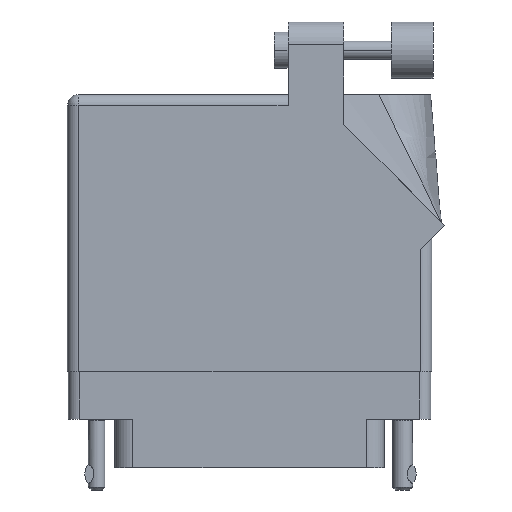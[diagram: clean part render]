
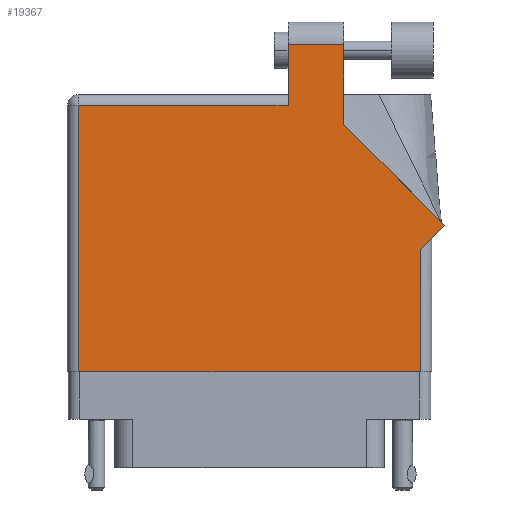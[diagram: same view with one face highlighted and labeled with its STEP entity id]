
A CAD part, front view. The second image highlights one B-rep face of the part: STEP entity #19367.
In plain terms, the highlighted face is planar.
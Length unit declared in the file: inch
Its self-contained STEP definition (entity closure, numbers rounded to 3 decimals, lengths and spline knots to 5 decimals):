
#991 = LINE ( 'NONE', #34836, #15941 ) ;
#2304 = LINE ( 'NONE', #2780, #33323 ) ;
#2695 = VECTOR ( 'NONE', #29667, 39.37008 ) ;
#2780 = CARTESIAN_POINT ( 'NONE',  ( 1.217, 1.805, 0. ) ) ;
#2812 = LINE ( 'NONE', #7174, #17338 ) ;
#3273 = CARTESIAN_POINT ( 'NONE',  ( 0.062, 0., 0. ) ) ;
#3282 = EDGE_CURVE ( 'NONE', #24721, #35827, #991, .T. ) ;
#3291 = DIRECTION ( 'NONE',  ( 0., 0., -1. ) ) ;
#3774 = LINE ( 'NONE', #36929, #26237 ) ;
#3916 = LINE ( 'NONE', #25343, #33777 ) ;
#4120 = VERTEX_POINT ( 'NONE', #3273 ) ;
#4923 = DIRECTION ( 'NONE',  ( 1., 0., 0. ) ) ;
#5076 = CARTESIAN_POINT ( 'NONE',  ( 0.062, 1.468, 0. ) ) ;
#5631 = CARTESIAN_POINT ( 'NONE',  ( 0., 0., 0. ) ) ;
#6454 = DIRECTION ( 'NONE',  ( 0., 1., 0. ) ) ;
#6923 = FACE_OUTER_BOUND ( 'NONE', #23280, .T. ) ;
#7174 = CARTESIAN_POINT ( 'NONE',  ( 1.948, 0.737, 0. ) ) ;
#8899 = EDGE_CURVE ( 'NONE', #35827, #4120, #3774, .T. ) ;
#9675 = ORIENTED_EDGE ( 'NONE', *, *, #13024, .T. ) ;
#10010 = ORIENTED_EDGE ( 'NONE', *, *, #8899, .T. ) ;
#10727 = CARTESIAN_POINT ( 'NONE',  ( 2.08071, 0.80771, 0. ) ) ;
#11122 = ORIENTED_EDGE ( 'NONE', *, *, #27927, .T. ) ;
#11162 = CARTESIAN_POINT ( 'NONE',  ( 1.217, 1.53, 0. ) ) ;
#11231 = VERTEX_POINT ( 'NONE', #44173 ) ;
#11460 = ORIENTED_EDGE ( 'NONE', *, *, #27510, .T. ) ;
#12189 = ORIENTED_EDGE ( 'NONE', *, *, #45232, .T. ) ;
#12215 = EDGE_CURVE ( 'NONE', #31965, #12978, #2304, .T. ) ;
#12978 = VERTEX_POINT ( 'NONE', #43767 ) ;
#13024 = EDGE_CURVE ( 'NONE', #14586, #31965, #15428, .T. ) ;
#14499 = DIRECTION ( 'NONE',  ( 0., -1., 0. ) ) ;
#14586 = VERTEX_POINT ( 'NONE', #27581 ) ;
#14892 = DIRECTION ( 'NONE',  ( -0.707, 0.707, 0. ) ) ;
#14960 = ORIENTED_EDGE ( 'NONE', *, *, #38919, .T. ) ;
#15428 = LINE ( 'NONE', #15677, #27166 ) ;
#15677 = CARTESIAN_POINT ( 'NONE',  ( 1.524, 1.36442, 0. ) ) ;
#15773 = CARTESIAN_POINT ( 'NONE',  ( 1.217, 1.468, 0. ) ) ;
#15941 = VECTOR ( 'NONE', #31177, 39.37008 ) ;
#17338 = VECTOR ( 'NONE', #6454, 39.37008 ) ;
#17502 = EDGE_CURVE ( 'NONE', #4120, #17729, #35360, .T. ) ;
#17729 = VERTEX_POINT ( 'NONE', #28741 ) ;
#18152 = DIRECTION ( 'NONE',  ( -1., 0., 0. ) ) ;
#19367 = ADVANCED_FACE ( 'NONE', ( #6923 ), #32274, .F. ) ;
#21389 = AXIS2_PLACEMENT_3D ( 'NONE', #47195, #3291, #18152 ) ;
#22924 = DIRECTION ( 'NONE',  ( 0.707, 0.707, 0. ) ) ;
#23280 = EDGE_LOOP ( 'NONE', ( #9675, #44128, #11122, #45093, #10010, #26977, #12189, #14960, #11460 ) ) ;
#24721 = VERTEX_POINT ( 'NONE', #15773 ) ;
#25343 = CARTESIAN_POINT ( 'NONE',  ( 2.08071, 0.80771, 0. ) ) ;
#26237 = VECTOR ( 'NONE', #14499, 39.37008 ) ;
#26573 = LINE ( 'NONE', #41479, #42913 ) ;
#26977 = ORIENTED_EDGE ( 'NONE', *, *, #17502, .T. ) ;
#27166 = VECTOR ( 'NONE', #44730, 39.37008 ) ;
#27510 = EDGE_CURVE ( 'NONE', #34818, #14586, #3916, .T. ) ;
#27581 = CARTESIAN_POINT ( 'NONE',  ( 1.524, 1.36442, 0. ) ) ;
#27927 = EDGE_CURVE ( 'NONE', #12978, #24721, #47750, .T. ) ;
#28741 = CARTESIAN_POINT ( 'NONE',  ( 1.948, 0., 0. ) ) ;
#29667 = DIRECTION ( 'NONE',  ( 0., -1., 0. ) ) ;
#31177 = DIRECTION ( 'NONE',  ( -1., 0., 0. ) ) ;
#31965 = VERTEX_POINT ( 'NONE', #38872 ) ;
#32274 = PLANE ( 'NONE',  #21389 ) ;
#33323 = VECTOR ( 'NONE', #40092, 39.37008 ) ;
#33777 = VECTOR ( 'NONE', #14892, 39.37008 ) ;
#34818 = VERTEX_POINT ( 'NONE', #10727 ) ;
#34836 = CARTESIAN_POINT ( 'NONE',  ( 0., 1.468, 0. ) ) ;
#35360 = LINE ( 'NONE', #5631, #40333 ) ;
#35827 = VERTEX_POINT ( 'NONE', #5076 ) ;
#36929 = CARTESIAN_POINT ( 'NONE',  ( 0.062, 0., 0. ) ) ;
#38872 = CARTESIAN_POINT ( 'NONE',  ( 1.524, 1.805, 0. ) ) ;
#38919 = EDGE_CURVE ( 'NONE', #11231, #34818, #26573, .T. ) ;
#40092 = DIRECTION ( 'NONE',  ( -1., 0., 0. ) ) ;
#40333 = VECTOR ( 'NONE', #4923, 39.37008 ) ;
#41479 = CARTESIAN_POINT ( 'NONE',  ( 2.01, 0.737, 0. ) ) ;
#42913 = VECTOR ( 'NONE', #22924, 39.37008 ) ;
#43767 = CARTESIAN_POINT ( 'NONE',  ( 1.217, 1.805, 0. ) ) ;
#44128 = ORIENTED_EDGE ( 'NONE', *, *, #12215, .T. ) ;
#44173 = CARTESIAN_POINT ( 'NONE',  ( 1.948, 0.675, 0. ) ) ;
#44730 = DIRECTION ( 'NONE',  ( 0., 1., 0. ) ) ;
#45093 = ORIENTED_EDGE ( 'NONE', *, *, #3282, .T. ) ;
#45232 = EDGE_CURVE ( 'NONE', #17729, #11231, #2812, .T. ) ;
#47195 = CARTESIAN_POINT ( 'NONE',  ( 0., 1.53, 0. ) ) ;
#47750 = LINE ( 'NONE', #11162, #2695 ) ;
